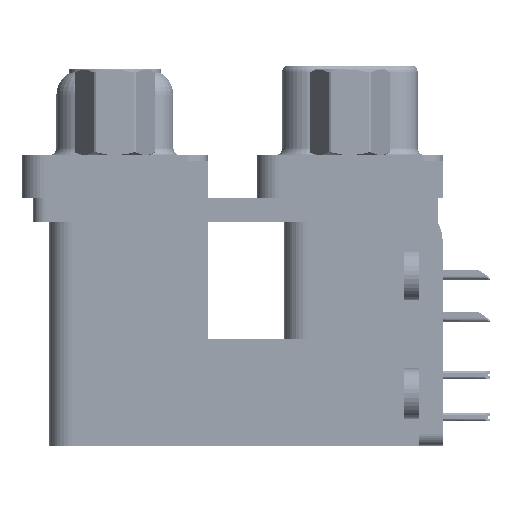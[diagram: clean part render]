
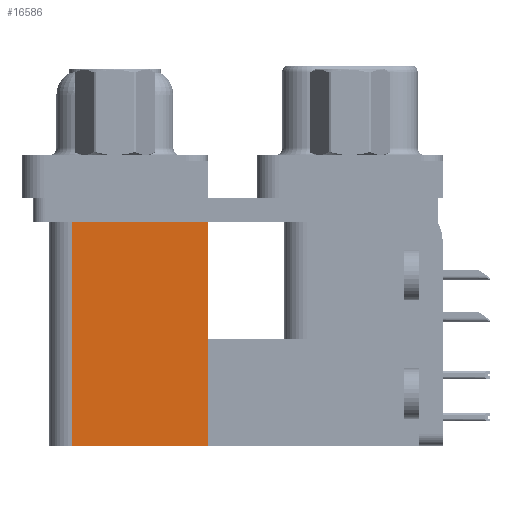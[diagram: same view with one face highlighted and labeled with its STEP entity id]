
A CAD part, left-side view. The second image highlights one B-rep face of the part: STEP entity #16586.
In plain terms, the highlighted planar face has unit normal (-1, 0, 0).
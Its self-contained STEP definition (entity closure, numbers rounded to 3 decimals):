
#326 = CARTESIAN_POINT ( 'NONE',  ( 3.79, 9.6, -19.2 ) ) ;
#1312 = CARTESIAN_POINT ( 'NONE',  ( 3.79, 18.8, -19.2 ) ) ;
#2363 = FACE_OUTER_BOUND ( 'NONE', #41471, .T. ) ;
#3336 = VECTOR ( 'NONE', #4853, 1000. ) ;
#4778 = CARTESIAN_POINT ( 'NONE',  ( 3.79, 18.8, -2.5 ) ) ;
#4853 = DIRECTION ( 'NONE',  ( 0., 0., 1. ) ) ;
#8484 = VECTOR ( 'NONE', #18799, 1000. ) ;
#8838 = ORIENTED_EDGE ( 'NONE', *, *, #51044, .F. ) ;
#13318 = LINE ( 'NONE', #42201, #16590 ) ;
#13367 = PLANE ( 'NONE',  #15442 ) ;
#15442 = AXIS2_PLACEMENT_3D ( 'NONE', #42628, #71789, #32007 ) ;
#16586 = ADVANCED_FACE ( 'NONE', ( #2363 ), #13367, .F. ) ;
#16590 = VECTOR ( 'NONE', #65325, 1000. ) ;
#18732 = VERTEX_POINT ( 'NONE', #4778 ) ;
#18799 = DIRECTION ( 'NONE',  ( 0., 1., 0. ) ) ;
#24893 = EDGE_CURVE ( 'NONE', #41392, #39682, #45159, .T. ) ;
#29811 = CARTESIAN_POINT ( 'NONE',  ( 3.79, 9.6, -19.2 ) ) ;
#30216 = EDGE_CURVE ( 'NONE', #39682, #18732, #13318, .T. ) ;
#32007 = DIRECTION ( 'NONE',  ( 0., 1., 0. ) ) ;
#33216 = EDGE_CURVE ( 'NONE', #41392, #38127, #70365, .T. ) ;
#38127 = VERTEX_POINT ( 'NONE', #1312 ) ;
#39682 = VERTEX_POINT ( 'NONE', #56702 ) ;
#41392 = VERTEX_POINT ( 'NONE', #49511 ) ;
#41471 = EDGE_LOOP ( 'NONE', ( #67552, #8838, #60573, #55329 ) ) ;
#42201 = CARTESIAN_POINT ( 'NONE',  ( 3.79, 9.6, -2.5 ) ) ;
#42628 = CARTESIAN_POINT ( 'NONE',  ( 3.79, 9.6, -19.2 ) ) ;
#45159 = LINE ( 'NONE', #326, #59859 ) ;
#49511 = CARTESIAN_POINT ( 'NONE',  ( 3.79, 9.6, -19.2 ) ) ;
#51044 = EDGE_CURVE ( 'NONE', #38127, #18732, #68239, .T. ) ;
#55329 = ORIENTED_EDGE ( 'NONE', *, *, #24893, .T. ) ;
#56702 = CARTESIAN_POINT ( 'NONE',  ( 3.79, 9.6, -2.5 ) ) ;
#56874 = CARTESIAN_POINT ( 'NONE',  ( 3.79, 18.8, -19.2 ) ) ;
#59859 = VECTOR ( 'NONE', #68256, 1000. ) ;
#60573 = ORIENTED_EDGE ( 'NONE', *, *, #33216, .F. ) ;
#65325 = DIRECTION ( 'NONE',  ( 0., 1., 0. ) ) ;
#67552 = ORIENTED_EDGE ( 'NONE', *, *, #30216, .T. ) ;
#68239 = LINE ( 'NONE', #56874, #3336 ) ;
#68256 = DIRECTION ( 'NONE',  ( 0., 0., 1. ) ) ;
#70365 = LINE ( 'NONE', #29811, #8484 ) ;
#71789 = DIRECTION ( 'NONE',  ( 1., 0., 0. ) ) ;
